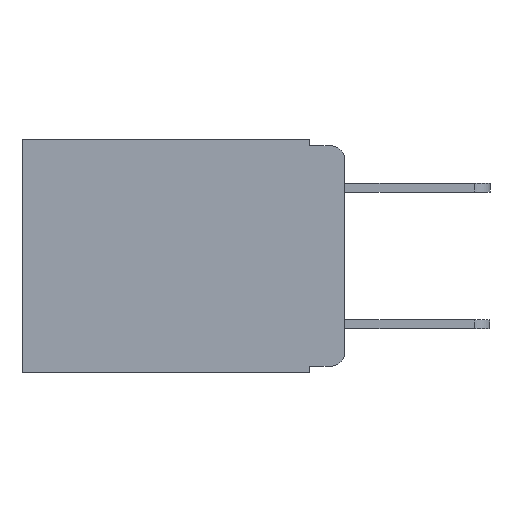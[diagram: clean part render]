
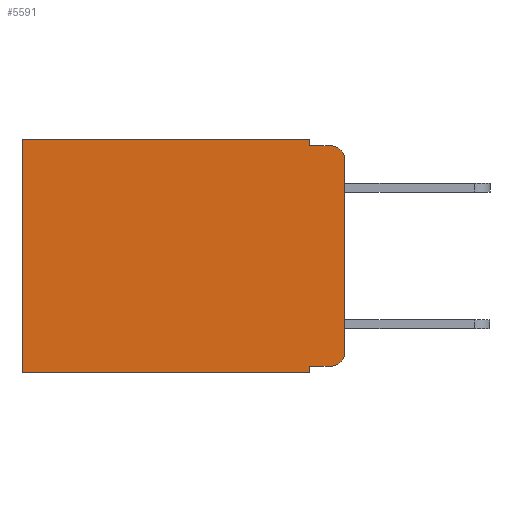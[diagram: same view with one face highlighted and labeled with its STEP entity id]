
A CAD part, left-side view. The second image highlights one B-rep face of the part: STEP entity #5591.
In plain terms, the highlighted planar face has unit normal (-1, 0, 0).
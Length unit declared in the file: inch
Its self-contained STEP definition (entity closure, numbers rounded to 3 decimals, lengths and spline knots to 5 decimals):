
#1 = CARTESIAN_POINT ( 'NONE',  ( 0.298, 0.051, -0.343 ) ) ;
#94 = DIRECTION ( 'NONE',  ( 0., 0., -1. ) ) ;
#137 = VERTEX_POINT ( 'NONE', #5199 ) ;
#174 = VERTEX_POINT ( 'NONE', #5819 ) ;
#247 = CARTESIAN_POINT ( 'NONE',  ( 0.298, 0.473, -0.343 ) ) ;
#323 = VERTEX_POINT ( 'NONE', #3847 ) ;
#586 = CARTESIAN_POINT ( 'NONE',  ( 0.298, 0.051, 0. ) ) ;
#604 = EDGE_CURVE ( 'NONE', #323, #5891, #3569, .T. ) ;
#697 = EDGE_CURVE ( 'NONE', #174, #7694, #2772, .T. ) ;
#824 = VERTEX_POINT ( 'NONE', #1519 ) ;
#835 = VERTEX_POINT ( 'NONE', #6115 ) ;
#864 = ORIENTED_EDGE ( 'NONE', *, *, #4937, .F. ) ;
#878 = ORIENTED_EDGE ( 'NONE', *, *, #8090, .T. ) ;
#1044 = LINE ( 'NONE', #8952, #9284 ) ;
#1187 = CIRCLE ( 'NONE', #4581, 0.02 ) ;
#1204 = PLANE ( 'NONE',  #9656 ) ;
#1519 = CARTESIAN_POINT ( 'NONE',  ( 0.298, 0., -0.313 ) ) ;
#2161 = VECTOR ( 'NONE', #3275, 39.37008 ) ;
#2216 = EDGE_CURVE ( 'NONE', #835, #5891, #1187, .T. ) ;
#2371 = ORIENTED_EDGE ( 'NONE', *, *, #4058, .F. ) ;
#2499 = VECTOR ( 'NONE', #7381, 39.37008 ) ;
#2604 = ORIENTED_EDGE ( 'NONE', *, *, #697, .T. ) ;
#2669 = EDGE_CURVE ( 'NONE', #7225, #137, #3910, .T. ) ;
#2772 = LINE ( 'NONE', #6975, #2499 ) ;
#3067 = DIRECTION ( 'NONE',  ( 0., 0., -1. ) ) ;
#3166 = DIRECTION ( 'NONE',  ( 0., 0., -1. ) ) ;
#3275 = DIRECTION ( 'NONE',  ( 0., 0., -1. ) ) ;
#3569 = LINE ( 'NONE', #7107, #9832 ) ;
#3627 = EDGE_CURVE ( 'NONE', #4077, #10126, #6491, .T. ) ;
#3847 = CARTESIAN_POINT ( 'NONE',  ( 0.298, 0.051, -0.01 ) ) ;
#3910 = LINE ( 'NONE', #7892, #10394 ) ;
#4056 = ORIENTED_EDGE ( 'NONE', *, *, #3627, .F. ) ;
#4058 = EDGE_CURVE ( 'NONE', #7225, #323, #6371, .T. ) ;
#4077 = VERTEX_POINT ( 'NONE', #1 ) ;
#4119 = LINE ( 'NONE', #8617, #8265 ) ;
#4228 = ORIENTED_EDGE ( 'NONE', *, *, #604, .F. ) ;
#4255 = VECTOR ( 'NONE', #5182, 39.37008 ) ;
#4289 = CARTESIAN_POINT ( 'NONE',  ( 0.298, 0.051, 0. ) ) ;
#4551 = DIRECTION ( 'NONE',  ( 1., 0., 0. ) ) ;
#4581 = AXIS2_PLACEMENT_3D ( 'NONE', #4845, #10499, #5692 ) ;
#4726 = EDGE_CURVE ( 'NONE', #7694, #824, #8386, .T. ) ;
#4845 = CARTESIAN_POINT ( 'NONE',  ( 0.298, 0.02, -0.03 ) ) ;
#4927 = ORIENTED_EDGE ( 'NONE', *, *, #4726, .T. ) ;
#4937 = EDGE_CURVE ( 'NONE', #835, #824, #4119, .T. ) ;
#5039 = DIRECTION ( 'NONE',  ( -1., 0., 0. ) ) ;
#5182 = DIRECTION ( 'NONE',  ( 0., 1., 0. ) ) ;
#5199 = CARTESIAN_POINT ( 'NONE',  ( 0.298, 0.473, 0. ) ) ;
#5344 = AXIS2_PLACEMENT_3D ( 'NONE', #9900, #5039, #94 ) ;
#5591 = ADVANCED_FACE ( 'NONE', ( #6199 ), #1204, .F. ) ;
#5692 = DIRECTION ( 'NONE',  ( 0., 0., -1. ) ) ;
#5819 = CARTESIAN_POINT ( 'NONE',  ( 0.298, 0.051, -0.333 ) ) ;
#5891 = VERTEX_POINT ( 'NONE', #7376 ) ;
#6115 = CARTESIAN_POINT ( 'NONE',  ( 0.298, 0., -0.03 ) ) ;
#6199 = FACE_OUTER_BOUND ( 'NONE', #9387, .T. ) ;
#6240 = DIRECTION ( 'NONE',  ( 0., 1., 0. ) ) ;
#6371 = LINE ( 'NONE', #9046, #2161 ) ;
#6491 = LINE ( 'NONE', #10028, #4255 ) ;
#6907 = EDGE_CURVE ( 'NONE', #174, #4077, #8848, .T. ) ;
#6975 = CARTESIAN_POINT ( 'NONE',  ( 0.298, 0.051, -0.333 ) ) ;
#7107 = CARTESIAN_POINT ( 'NONE',  ( 0.298, 0.051, -0.01 ) ) ;
#7225 = VERTEX_POINT ( 'NONE', #4289 ) ;
#7376 = CARTESIAN_POINT ( 'NONE',  ( 0.298, 0.02, -0.01 ) ) ;
#7381 = DIRECTION ( 'NONE',  ( 0., -1., 0. ) ) ;
#7494 = ORIENTED_EDGE ( 'NONE', *, *, #2216, .T. ) ;
#7694 = VERTEX_POINT ( 'NONE', #8424 ) ;
#7892 = CARTESIAN_POINT ( 'NONE',  ( 0.298, 0., 0. ) ) ;
#8090 = EDGE_CURVE ( 'NONE', #137, #10126, #1044, .T. ) ;
#8265 = VECTOR ( 'NONE', #9397, 39.37008 ) ;
#8386 = CIRCLE ( 'NONE', #5344, 0.02 ) ;
#8424 = CARTESIAN_POINT ( 'NONE',  ( 0.298, 0.02, -0.333 ) ) ;
#8617 = CARTESIAN_POINT ( 'NONE',  ( 0.298, 0., 0. ) ) ;
#8848 = LINE ( 'NONE', #586, #10416 ) ;
#8952 = CARTESIAN_POINT ( 'NONE',  ( 0.298, 0.473, 0. ) ) ;
#9046 = CARTESIAN_POINT ( 'NONE',  ( 0.298, 0.051, 0. ) ) ;
#9284 = VECTOR ( 'NONE', #3166, 39.37008 ) ;
#9368 = ORIENTED_EDGE ( 'NONE', *, *, #2669, .T. ) ;
#9387 = EDGE_LOOP ( 'NONE', ( #864, #7494, #4228, #2371, #9368, #878, #4056, #9939, #2604, #4927 ) ) ;
#9397 = DIRECTION ( 'NONE',  ( 0., 0., -1. ) ) ;
#9440 = CARTESIAN_POINT ( 'NONE',  ( 0.298, 0., 0. ) ) ;
#9656 = AXIS2_PLACEMENT_3D ( 'NONE', #9440, #4551, #10242 ) ;
#9787 = DIRECTION ( 'NONE',  ( 0., -1., 0. ) ) ;
#9832 = VECTOR ( 'NONE', #9787, 39.37008 ) ;
#9900 = CARTESIAN_POINT ( 'NONE',  ( 0.298, 0.02, -0.313 ) ) ;
#9939 = ORIENTED_EDGE ( 'NONE', *, *, #6907, .F. ) ;
#10028 = CARTESIAN_POINT ( 'NONE',  ( 0.298, 0., -0.343 ) ) ;
#10126 = VERTEX_POINT ( 'NONE', #247 ) ;
#10242 = DIRECTION ( 'NONE',  ( 0., 0., -1. ) ) ;
#10394 = VECTOR ( 'NONE', #6240, 39.37008 ) ;
#10416 = VECTOR ( 'NONE', #3067, 39.37008 ) ;
#10499 = DIRECTION ( 'NONE',  ( -1., 0., 0. ) ) ;
